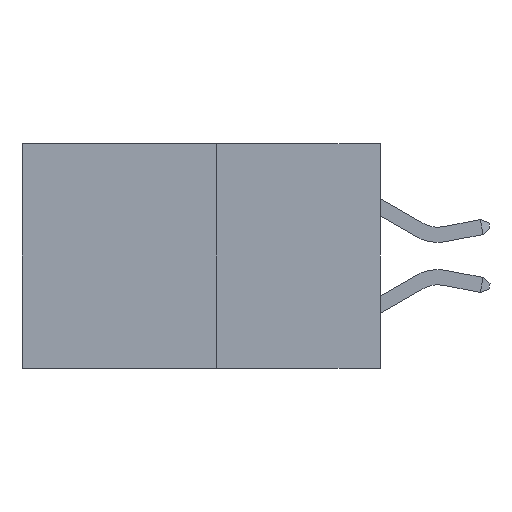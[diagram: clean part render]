
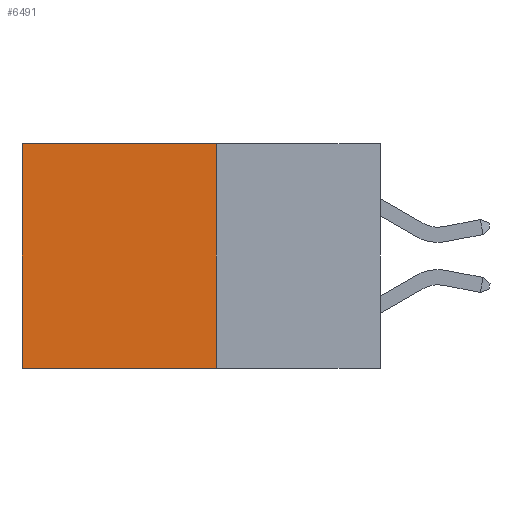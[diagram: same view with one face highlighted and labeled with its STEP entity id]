
A CAD part, left-side view. The second image highlights one B-rep face of the part: STEP entity #6491.
In plain terms, the highlighted planar face has unit normal (-1, 0, 0).
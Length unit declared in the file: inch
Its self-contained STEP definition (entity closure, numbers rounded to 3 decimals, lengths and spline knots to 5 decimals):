
#171 = CARTESIAN_POINT ( 'NONE',  ( 0.277, 0.59, -0.37 ) ) ;
#188 = DIRECTION ( 'NONE',  ( 0., 1., 0. ) ) ;
#548 = ORIENTED_EDGE ( 'NONE', *, *, #7066, .T. ) ;
#661 = EDGE_CURVE ( 'NONE', #694, #4399, #1295, .T. ) ;
#694 = VERTEX_POINT ( 'NONE', #2293 ) ;
#867 = LINE ( 'NONE', #3536, #5649 ) ;
#873 = CARTESIAN_POINT ( 'NONE',  ( 0.277, 0.27, -0.37 ) ) ;
#1295 = LINE ( 'NONE', #7319, #4634 ) ;
#1389 = EDGE_LOOP ( 'NONE', ( #548, #3021, #2970, #2926 ) ) ;
#1393 = DIRECTION ( 'NONE',  ( 0., 0., -1. ) ) ;
#1497 = DIRECTION ( 'NONE',  ( 0., 0., -1. ) ) ;
#2037 = FACE_OUTER_BOUND ( 'NONE', #1389, .T. ) ;
#2068 = CARTESIAN_POINT ( 'NONE',  ( 0.277, 0.27, 0. ) ) ;
#2149 = VERTEX_POINT ( 'NONE', #4253 ) ;
#2293 = CARTESIAN_POINT ( 'NONE',  ( 0.277, 0.27, 0. ) ) ;
#2837 = AXIS2_PLACEMENT_3D ( 'NONE', #873, #5243, #1497 ) ;
#2926 = ORIENTED_EDGE ( 'NONE', *, *, #5146, .T. ) ;
#2970 = ORIENTED_EDGE ( 'NONE', *, *, #661, .F. ) ;
#3021 = ORIENTED_EDGE ( 'NONE', *, *, #6655, .F. ) ;
#3093 = VECTOR ( 'NONE', #1393, 39.37008 ) ;
#3536 = CARTESIAN_POINT ( 'NONE',  ( 0.277, 0.27, -0.37 ) ) ;
#3999 = VECTOR ( 'NONE', #188, 39.37008 ) ;
#4175 = DIRECTION ( 'NONE',  ( 0., 1., 0. ) ) ;
#4253 = CARTESIAN_POINT ( 'NONE',  ( 0.277, 0.59, 0. ) ) ;
#4399 = VERTEX_POINT ( 'NONE', #6696 ) ;
#4587 = LINE ( 'NONE', #7050, #3093 ) ;
#4634 = VECTOR ( 'NONE', #7297, 39.37008 ) ;
#5146 = EDGE_CURVE ( 'NONE', #694, #2149, #5658, .T. ) ;
#5243 = DIRECTION ( 'NONE',  ( 1., 0., 0. ) ) ;
#5649 = VECTOR ( 'NONE', #4175, 39.37008 ) ;
#5658 = LINE ( 'NONE', #2068, #3999 ) ;
#6437 = VERTEX_POINT ( 'NONE', #171 ) ;
#6491 = ADVANCED_FACE ( 'NONE', ( #2037 ), #7687, .F. ) ;
#6655 = EDGE_CURVE ( 'NONE', #4399, #6437, #867, .T. ) ;
#6696 = CARTESIAN_POINT ( 'NONE',  ( 0.277, 0.27, -0.37 ) ) ;
#7050 = CARTESIAN_POINT ( 'NONE',  ( 0.277, 0.59, -0.37 ) ) ;
#7066 = EDGE_CURVE ( 'NONE', #2149, #6437, #4587, .T. ) ;
#7297 = DIRECTION ( 'NONE',  ( 0., 0., -1. ) ) ;
#7319 = CARTESIAN_POINT ( 'NONE',  ( 0.277, 0.27, -0.37 ) ) ;
#7687 = PLANE ( 'NONE',  #2837 ) ;
